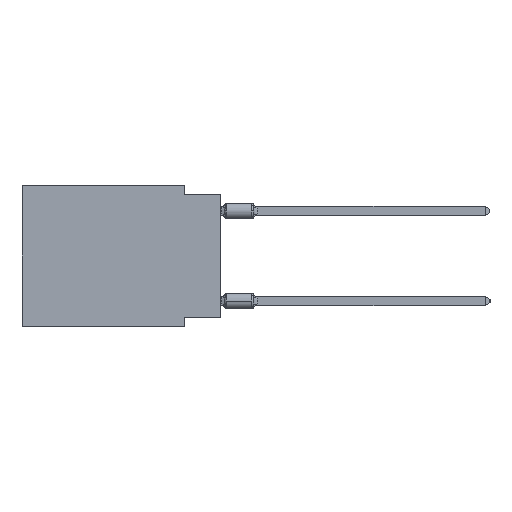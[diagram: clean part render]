
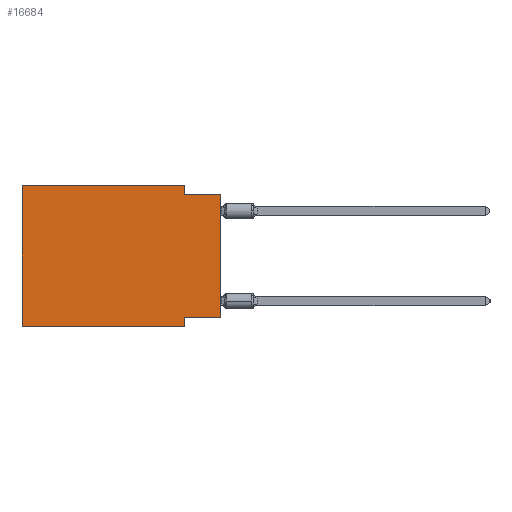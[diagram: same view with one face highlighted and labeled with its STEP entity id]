
A CAD part, left-side view. The second image highlights one B-rep face of the part: STEP entity #16684.
In plain terms, the highlighted planar face has unit normal (-1, 0, 0).
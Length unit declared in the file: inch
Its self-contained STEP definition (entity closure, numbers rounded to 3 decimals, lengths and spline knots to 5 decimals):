
#385 = VECTOR ( 'NONE', #9927, 39.37008 ) ;
#1032 = VECTOR ( 'NONE', #24667, 39.37008 ) ;
#1299 = CARTESIAN_POINT ( 'NONE',  ( 0., 0.55, 0. ) ) ;
#2086 = VECTOR ( 'NONE', #11603, 39.37008 ) ;
#2271 = CARTESIAN_POINT ( 'NONE',  ( 0., 0., -0.365 ) ) ;
#2514 = VECTOR ( 'NONE', #4278, 39.37008 ) ;
#2638 = ORIENTED_EDGE ( 'NONE', *, *, #16402, .F. ) ;
#2846 = VERTEX_POINT ( 'NONE', #12685 ) ;
#3281 = LINE ( 'NONE', #13587, #17244 ) ;
#4278 = DIRECTION ( 'NONE',  ( 0., 0., -1. ) ) ;
#4667 = CARTESIAN_POINT ( 'NONE',  ( 0., 0.55, 0. ) ) ;
#4895 = LINE ( 'NONE', #8153, #20918 ) ;
#5333 = ORIENTED_EDGE ( 'NONE', *, *, #14929, .F. ) ;
#5405 = PLANE ( 'NONE',  #12544 ) ;
#6284 = CARTESIAN_POINT ( 'NONE',  ( 0., 0.55, -0.39 ) ) ;
#6437 = ORIENTED_EDGE ( 'NONE', *, *, #17038, .F. ) ;
#6940 = DIRECTION ( 'NONE',  ( 0., 1., 0. ) ) ;
#7521 = LINE ( 'NONE', #10427, #385 ) ;
#7802 = VERTEX_POINT ( 'NONE', #2271 ) ;
#8153 = CARTESIAN_POINT ( 'NONE',  ( 0., 0., 0. ) ) ;
#8177 = VECTOR ( 'NONE', #27076, 39.37008 ) ;
#9302 = CARTESIAN_POINT ( 'NONE',  ( 0., 0., -0.025 ) ) ;
#9927 = DIRECTION ( 'NONE',  ( 0., -1., 0. ) ) ;
#10427 = CARTESIAN_POINT ( 'NONE',  ( 0., 0., -0.025 ) ) ;
#10711 = DIRECTION ( 'NONE',  ( 0., 0., 1. ) ) ;
#10721 = DIRECTION ( 'NONE',  ( 0., 0., -1. ) ) ;
#11015 = ORIENTED_EDGE ( 'NONE', *, *, #20164, .T. ) ;
#11603 = DIRECTION ( 'NONE',  ( 0., 0., 1. ) ) ;
#12121 = LINE ( 'NONE', #1299, #2086 ) ;
#12544 = AXIS2_PLACEMENT_3D ( 'NONE', #21549, #24138, #10721 ) ;
#12685 = CARTESIAN_POINT ( 'NONE',  ( 0., 0.1, 0. ) ) ;
#13587 = CARTESIAN_POINT ( 'NONE',  ( 0., 0.55, 0. ) ) ;
#13758 = DIRECTION ( 'NONE',  ( 0., -1., 0. ) ) ;
#14929 = EDGE_CURVE ( 'NONE', #29391, #26525, #7521, .T. ) ;
#15428 = ORIENTED_EDGE ( 'NONE', *, *, #32033, .T. ) ;
#15874 = FACE_OUTER_BOUND ( 'NONE', #20333, .T. ) ;
#16402 = EDGE_CURVE ( 'NONE', #26187, #29690, #12121, .T. ) ;
#16684 = ADVANCED_FACE ( 'NONE', ( #15874 ), #5405, .F. ) ;
#16743 = CARTESIAN_POINT ( 'NONE',  ( 0., 0.1, -0.39 ) ) ;
#16891 = CARTESIAN_POINT ( 'NONE',  ( 0., 0., -0.365 ) ) ;
#17038 = EDGE_CURVE ( 'NONE', #24493, #22949, #33062, .T. ) ;
#17116 = CARTESIAN_POINT ( 'NONE',  ( 0., 0.55, -0.39 ) ) ;
#17244 = VECTOR ( 'NONE', #13758, 39.37008 ) ;
#17785 = ORIENTED_EDGE ( 'NONE', *, *, #23517, .F. ) ;
#18293 = VECTOR ( 'NONE', #6940, 39.37008 ) ;
#18981 = LINE ( 'NONE', #6284, #8177 ) ;
#20164 = EDGE_CURVE ( 'NONE', #7802, #26525, #4895, .T. ) ;
#20333 = EDGE_LOOP ( 'NONE', ( #11015, #5333, #32372, #33663, #2638, #15428, #6437, #17785 ) ) ;
#20564 = LINE ( 'NONE', #22644, #2514 ) ;
#20918 = VECTOR ( 'NONE', #10711, 39.37008 ) ;
#21549 = CARTESIAN_POINT ( 'NONE',  ( 0., 0.55, 0. ) ) ;
#21750 = CARTESIAN_POINT ( 'NONE',  ( 0., 0.1, -0.39 ) ) ;
#22560 = LINE ( 'NONE', #16891, #18293 ) ;
#22644 = CARTESIAN_POINT ( 'NONE',  ( 0., 0.1, 0. ) ) ;
#22949 = VERTEX_POINT ( 'NONE', #21750 ) ;
#23517 = EDGE_CURVE ( 'NONE', #7802, #24493, #22560, .T. ) ;
#24138 = DIRECTION ( 'NONE',  ( 1., 0., 0. ) ) ;
#24493 = VERTEX_POINT ( 'NONE', #27484 ) ;
#24667 = DIRECTION ( 'NONE',  ( 0., 0., -1. ) ) ;
#25094 = EDGE_CURVE ( 'NONE', #29690, #2846, #3281, .T. ) ;
#26182 = CARTESIAN_POINT ( 'NONE',  ( 0., 0.1, -0.025 ) ) ;
#26187 = VERTEX_POINT ( 'NONE', #17116 ) ;
#26525 = VERTEX_POINT ( 'NONE', #9302 ) ;
#26963 = EDGE_CURVE ( 'NONE', #2846, #29391, #20564, .T. ) ;
#27076 = DIRECTION ( 'NONE',  ( 0., -1., 0. ) ) ;
#27484 = CARTESIAN_POINT ( 'NONE',  ( 0., 0.1, -0.365 ) ) ;
#29391 = VERTEX_POINT ( 'NONE', #26182 ) ;
#29690 = VERTEX_POINT ( 'NONE', #4667 ) ;
#32033 = EDGE_CURVE ( 'NONE', #26187, #22949, #18981, .T. ) ;
#32372 = ORIENTED_EDGE ( 'NONE', *, *, #26963, .F. ) ;
#33062 = LINE ( 'NONE', #16743, #1032 ) ;
#33663 = ORIENTED_EDGE ( 'NONE', *, *, #25094, .F. ) ;
